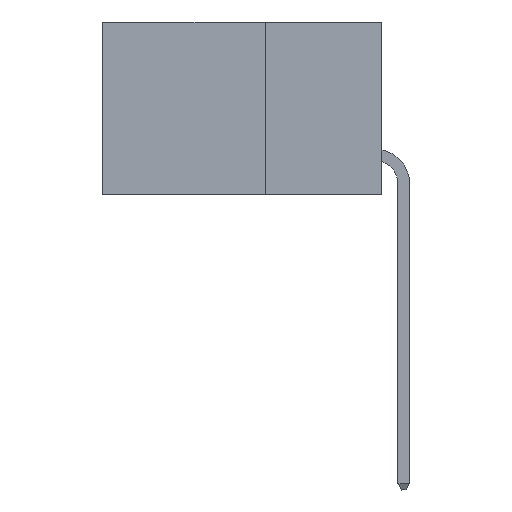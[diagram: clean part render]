
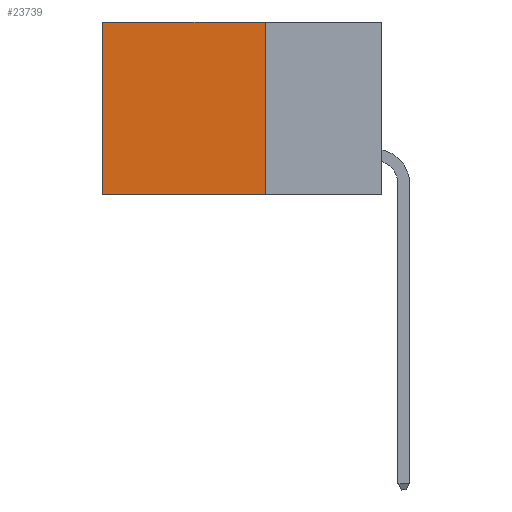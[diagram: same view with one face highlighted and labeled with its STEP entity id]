
A CAD part, left-side view. The second image highlights one B-rep face of the part: STEP entity #23739.
In plain terms, the highlighted planar face has unit normal (-1, 0, 0).
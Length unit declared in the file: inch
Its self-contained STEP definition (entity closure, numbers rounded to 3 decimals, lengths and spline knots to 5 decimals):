
#1783 = ORIENTED_EDGE ( 'NONE', *, *, #24046, .F. ) ;
#2044 = ORIENTED_EDGE ( 'NONE', *, *, #15946, .F. ) ;
#2957 = DIRECTION ( 'NONE',  ( 0., 1., 0. ) ) ;
#5584 = ORIENTED_EDGE ( 'NONE', *, *, #28152, .T. ) ;
#5689 = VECTOR ( 'NONE', #32398, 39.37008 ) ;
#7711 = CARTESIAN_POINT ( 'NONE',  ( 0.2875, 0.25, 0. ) ) ;
#7942 = CARTESIAN_POINT ( 'NONE',  ( 0.2875, 0.25, 0. ) ) ;
#8555 = CARTESIAN_POINT ( 'NONE',  ( 0.2875, 0.25, -0.37 ) ) ;
#9375 = VERTEX_POINT ( 'NONE', #8555 ) ;
#10790 = LINE ( 'NONE', #27504, #19760 ) ;
#13048 = LINE ( 'NONE', #7942, #5689 ) ;
#13116 = PLANE ( 'NONE',  #24590 ) ;
#15260 = EDGE_LOOP ( 'NONE', ( #5584, #2044, #1783, #16019 ) ) ;
#15946 = EDGE_CURVE ( 'NONE', #9375, #34574, #18185, .T. ) ;
#16019 = ORIENTED_EDGE ( 'NONE', *, *, #25207, .T. ) ;
#18185 = LINE ( 'NONE', #23768, #30484 ) ;
#19760 = VECTOR ( 'NONE', #2957, 39.37008 ) ;
#21260 = DIRECTION ( 'NONE',  ( 0., 0., -1. ) ) ;
#22403 = DIRECTION ( 'NONE',  ( 0., 0., -1. ) ) ;
#23649 = DIRECTION ( 'NONE',  ( 0., 1., 0. ) ) ;
#23739 = ADVANCED_FACE ( 'NONE', ( #29689 ), #13116, .F. ) ;
#23768 = CARTESIAN_POINT ( 'NONE',  ( 0.2875, 0.25, -0.37 ) ) ;
#23775 = CARTESIAN_POINT ( 'NONE',  ( 0.2875, 0.6, 0. ) ) ;
#24046 = EDGE_CURVE ( 'NONE', #35147, #9375, #13048, .T. ) ;
#24590 = AXIS2_PLACEMENT_3D ( 'NONE', #7711, #35057, #21260 ) ;
#25149 = CARTESIAN_POINT ( 'NONE',  ( 0.2875, 0.6, 0. ) ) ;
#25207 = EDGE_CURVE ( 'NONE', #35147, #30577, #10790, .T. ) ;
#25605 = CARTESIAN_POINT ( 'NONE',  ( 0.2875, 0.25, 0. ) ) ;
#27504 = CARTESIAN_POINT ( 'NONE',  ( 0.2875, 0.25, 0. ) ) ;
#28152 = EDGE_CURVE ( 'NONE', #30577, #34574, #32242, .T. ) ;
#29689 = FACE_OUTER_BOUND ( 'NONE', #15260, .T. ) ;
#30484 = VECTOR ( 'NONE', #23649, 39.37008 ) ;
#30577 = VERTEX_POINT ( 'NONE', #23775 ) ;
#31740 = VECTOR ( 'NONE', #22403, 39.37008 ) ;
#32242 = LINE ( 'NONE', #25149, #31740 ) ;
#32398 = DIRECTION ( 'NONE',  ( 0., 0., -1. ) ) ;
#34574 = VERTEX_POINT ( 'NONE', #34667 ) ;
#34667 = CARTESIAN_POINT ( 'NONE',  ( 0.2875, 0.6, -0.37 ) ) ;
#35057 = DIRECTION ( 'NONE',  ( 1., 0., 0. ) ) ;
#35147 = VERTEX_POINT ( 'NONE', #25605 ) ;
